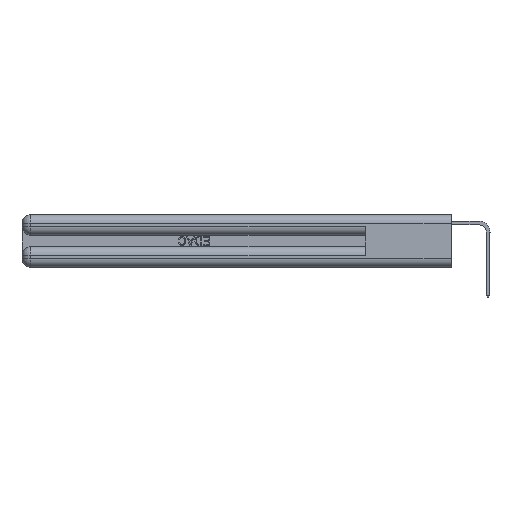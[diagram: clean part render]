
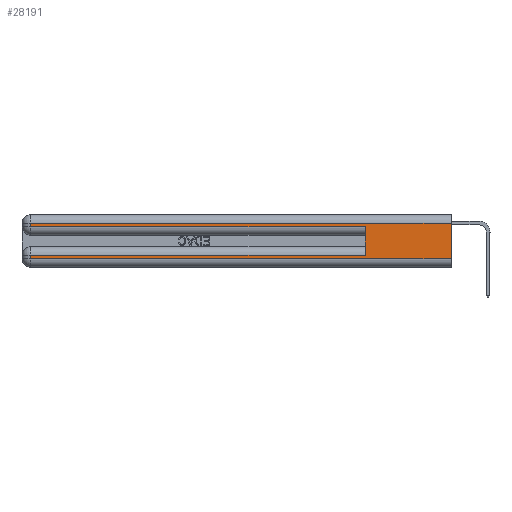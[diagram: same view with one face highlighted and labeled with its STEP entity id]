
A CAD part, left-side view. The second image highlights one B-rep face of the part: STEP entity #28191.
In plain terms, the highlighted planar face has unit normal (-1, 0, 0).
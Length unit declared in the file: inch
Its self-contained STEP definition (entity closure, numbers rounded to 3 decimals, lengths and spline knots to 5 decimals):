
#260 = LINE ( 'NONE', #2965, #5653 ) ;
#434 = ORIENTED_EDGE ( 'NONE', *, *, #9587, .T. ) ;
#1150 = DIRECTION ( 'NONE',  ( 0., 0., 1. ) ) ;
#1613 = ORIENTED_EDGE ( 'NONE', *, *, #3548, .F. ) ;
#2965 = CARTESIAN_POINT ( 'NONE',  ( 0., 0., 0.31 ) ) ;
#3076 = LINE ( 'NONE', #7576, #31258 ) ;
#3534 = CARTESIAN_POINT ( 'NONE',  ( 0., 2.94, 0.31 ) ) ;
#3548 = EDGE_CURVE ( 'NONE', #28564, #9433, #18901, .T. ) ;
#3614 = VERTEX_POINT ( 'NONE', #31488 ) ;
#4269 = CARTESIAN_POINT ( 'NONE',  ( 0., 2.94, 0.37 ) ) ;
#4640 = DIRECTION ( 'NONE',  ( 0., -1., 0. ) ) ;
#5082 = DIRECTION ( 'NONE',  ( 0., 1., 0. ) ) ;
#5589 = PLANE ( 'NONE',  #24753 ) ;
#5653 = VECTOR ( 'NONE', #16319, 39.37008 ) ;
#5716 = FACE_OUTER_BOUND ( 'NONE', #26300, .T. ) ;
#5822 = VECTOR ( 'NONE', #4640, 39.37008 ) ;
#7576 = CARTESIAN_POINT ( 'NONE',  ( 0., 2.94, 0.37 ) ) ;
#8021 = LINE ( 'NONE', #4269, #29098 ) ;
#9416 = CARTESIAN_POINT ( 'NONE',  ( 0., 0., 0.285 ) ) ;
#9433 = VERTEX_POINT ( 'NONE', #27809 ) ;
#9587 = EDGE_CURVE ( 'NONE', #29237, #14174, #3076, .T. ) ;
#10249 = EDGE_CURVE ( 'NONE', #13702, #20132, #32076, .T. ) ;
#10448 = ORIENTED_EDGE ( 'NONE', *, *, #33907, .T. ) ;
#10912 = DIRECTION ( 'NONE',  ( 0., 0., -1. ) ) ;
#11849 = VECTOR ( 'NONE', #1150, 39.37008 ) ;
#12556 = LINE ( 'NONE', #9416, #32803 ) ;
#12636 = CARTESIAN_POINT ( 'NONE',  ( 0., 0., 0.06 ) ) ;
#13350 = CARTESIAN_POINT ( 'NONE',  ( 0., 0.6, 0.085 ) ) ;
#13702 = VERTEX_POINT ( 'NONE', #13350 ) ;
#14174 = VERTEX_POINT ( 'NONE', #20494 ) ;
#14826 = DIRECTION ( 'NONE',  ( 0., 0., -1. ) ) ;
#15641 = CARTESIAN_POINT ( 'NONE',  ( 0., 0., 0.085 ) ) ;
#16319 = DIRECTION ( 'NONE',  ( 0., 1., 0. ) ) ;
#17037 = CARTESIAN_POINT ( 'NONE',  ( 0., 0.6, 0.145 ) ) ;
#17059 = ORIENTED_EDGE ( 'NONE', *, *, #33290, .T. ) ;
#18068 = LINE ( 'NONE', #17037, #11849 ) ;
#18088 = VECTOR ( 'NONE', #31262, 39.37008 ) ;
#18901 = LINE ( 'NONE', #23318, #18088 ) ;
#19053 = LINE ( 'NONE', #12636, #5822 ) ;
#19126 = ORIENTED_EDGE ( 'NONE', *, *, #26862, .T. ) ;
#20132 = VERTEX_POINT ( 'NONE', #32458 ) ;
#20494 = CARTESIAN_POINT ( 'NONE',  ( 0., 2.94, 0.285 ) ) ;
#22603 = DIRECTION ( 'NONE',  ( 0., -1., 0. ) ) ;
#23318 = CARTESIAN_POINT ( 'NONE',  ( 0., 0., 0.37 ) ) ;
#23709 = ORIENTED_EDGE ( 'NONE', *, *, #10249, .T. ) ;
#24104 = CARTESIAN_POINT ( 'NONE',  ( 0., 0., 0.37 ) ) ;
#24233 = VECTOR ( 'NONE', #5082, 39.37008 ) ;
#24453 = ORIENTED_EDGE ( 'NONE', *, *, #29076, .T. ) ;
#24753 = AXIS2_PLACEMENT_3D ( 'NONE', #24104, #26767, #10912 ) ;
#26085 = DIRECTION ( 'NONE',  ( 0., 0., -1. ) ) ;
#26300 = EDGE_LOOP ( 'NONE', ( #1613, #24453, #434, #17059, #29056, #23709, #10448, #19126 ) ) ;
#26767 = DIRECTION ( 'NONE',  ( 1., 0., 0. ) ) ;
#26862 = EDGE_CURVE ( 'NONE', #3614, #9433, #19053, .T. ) ;
#27809 = CARTESIAN_POINT ( 'NONE',  ( 0., 0., 0.06 ) ) ;
#28191 = ADVANCED_FACE ( 'NONE', ( #5716 ), #5589, .F. ) ;
#28564 = VERTEX_POINT ( 'NONE', #29974 ) ;
#29056 = ORIENTED_EDGE ( 'NONE', *, *, #31505, .F. ) ;
#29076 = EDGE_CURVE ( 'NONE', #28564, #29237, #260, .T. ) ;
#29098 = VECTOR ( 'NONE', #14826, 39.37008 ) ;
#29237 = VERTEX_POINT ( 'NONE', #3534 ) ;
#29528 = VERTEX_POINT ( 'NONE', #31198 ) ;
#29974 = CARTESIAN_POINT ( 'NONE',  ( 0., 0., 0.31 ) ) ;
#31198 = CARTESIAN_POINT ( 'NONE',  ( 0., 0.6, 0.285 ) ) ;
#31258 = VECTOR ( 'NONE', #26085, 39.37008 ) ;
#31262 = DIRECTION ( 'NONE',  ( 0., 0., -1. ) ) ;
#31488 = CARTESIAN_POINT ( 'NONE',  ( 0., 2.94, 0.06 ) ) ;
#31505 = EDGE_CURVE ( 'NONE', #13702, #29528, #18068, .T. ) ;
#32076 = LINE ( 'NONE', #15641, #24233 ) ;
#32458 = CARTESIAN_POINT ( 'NONE',  ( 0., 2.94, 0.085 ) ) ;
#32803 = VECTOR ( 'NONE', #22603, 39.37008 ) ;
#33290 = EDGE_CURVE ( 'NONE', #14174, #29528, #12556, .T. ) ;
#33907 = EDGE_CURVE ( 'NONE', #20132, #3614, #8021, .T. ) ;
